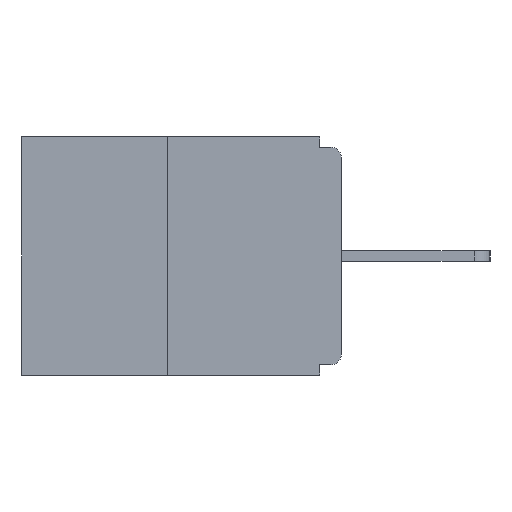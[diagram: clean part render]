
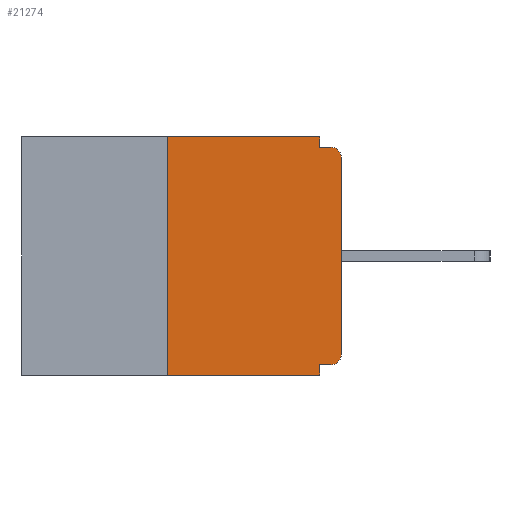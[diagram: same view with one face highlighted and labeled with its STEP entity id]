
A CAD part, left-side view. The second image highlights one B-rep face of the part: STEP entity #21274.
In plain terms, the highlighted planar face has unit normal (-1, 0, 0).
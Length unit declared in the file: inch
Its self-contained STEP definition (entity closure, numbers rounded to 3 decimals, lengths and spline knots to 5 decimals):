
#655 = VERTEX_POINT ( 'NONE', #2800 ) ;
#684 = LINE ( 'NONE', #15329, #5969 ) ;
#745 = LINE ( 'NONE', #10344, #6030 ) ;
#1100 = ORIENTED_EDGE ( 'NONE', *, *, #23193, .F. ) ;
#1425 = ORIENTED_EDGE ( 'NONE', *, *, #22198, .T. ) ;
#1452 = PLANE ( 'NONE',  #21890 ) ;
#1503 = VECTOR ( 'NONE', #11871, 39.37008 ) ;
#1712 = DIRECTION ( 'NONE',  ( 0., -1., 0. ) ) ;
#1864 = DIRECTION ( 'NONE',  ( 0., -1., 0. ) ) ;
#2619 = VECTOR ( 'NONE', #17987, 39.37008 ) ;
#2800 = CARTESIAN_POINT ( 'NONE',  ( 0., 0.25, 0. ) ) ;
#3467 = DIRECTION ( 'NONE',  ( 0., 0., -1. ) ) ;
#3542 = VERTEX_POINT ( 'NONE', #7040 ) ;
#3917 = FACE_OUTER_BOUND ( 'NONE', #17528, .T. ) ;
#4743 = VERTEX_POINT ( 'NONE', #6163 ) ;
#4797 = VECTOR ( 'NONE', #16912, 39.37008 ) ;
#4858 = CARTESIAN_POINT ( 'NONE',  ( 0., 0.031, -0.343 ) ) ;
#4873 = CARTESIAN_POINT ( 'NONE',  ( 0., 0.46, -0.343 ) ) ;
#5411 = EDGE_CURVE ( 'NONE', #11106, #9800, #15516, .T. ) ;
#5480 = VECTOR ( 'NONE', #18613, 39.37008 ) ;
#5969 = VECTOR ( 'NONE', #1712, 39.37008 ) ;
#6030 = VECTOR ( 'NONE', #12242, 39.37008 ) ;
#6163 = CARTESIAN_POINT ( 'NONE',  ( 0., 0.25, -0.343 ) ) ;
#6356 = LINE ( 'NONE', #24986, #11791 ) ;
#7040 = CARTESIAN_POINT ( 'NONE',  ( 0., 0.031, -0.328 ) ) ;
#7148 = VERTEX_POINT ( 'NONE', #17537 ) ;
#7246 = CARTESIAN_POINT ( 'NONE',  ( 0., 0.25, 0. ) ) ;
#7995 = CARTESIAN_POINT ( 'NONE',  ( 0., 0., -0.328 ) ) ;
#8064 = EDGE_CURVE ( 'NONE', #21727, #9620, #14606, .T. ) ;
#8852 = DIRECTION ( 'NONE',  ( 0., -1., 0. ) ) ;
#9620 = VERTEX_POINT ( 'NONE', #10226 ) ;
#9800 = VERTEX_POINT ( 'NONE', #14513 ) ;
#10187 = CARTESIAN_POINT ( 'NONE',  ( 0., 0.015, -0.03 ) ) ;
#10226 = CARTESIAN_POINT ( 'NONE',  ( 0., 0., -0.313 ) ) ;
#10344 = CARTESIAN_POINT ( 'NONE',  ( 0., 0.031, -0.343 ) ) ;
#10692 = EDGE_CURVE ( 'NONE', #14422, #9800, #6356, .T. ) ;
#10988 = CARTESIAN_POINT ( 'NONE',  ( 0., 0.015, -0.313 ) ) ;
#11106 = VERTEX_POINT ( 'NONE', #12963 ) ;
#11791 = VECTOR ( 'NONE', #1864, 39.37008 ) ;
#11871 = DIRECTION ( 'NONE',  ( 0., 1., 0. ) ) ;
#11885 = LINE ( 'NONE', #12737, #5480 ) ;
#12081 = DIRECTION ( 'NONE',  ( 0., 0., -1. ) ) ;
#12242 = DIRECTION ( 'NONE',  ( 0., 0., -1. ) ) ;
#12737 = CARTESIAN_POINT ( 'NONE',  ( 0., 0.031, 0. ) ) ;
#12838 = VERTEX_POINT ( 'NONE', #4858 ) ;
#12882 = DIRECTION ( 'NONE',  ( 0., 0., -1. ) ) ;
#12963 = CARTESIAN_POINT ( 'NONE',  ( 0., 0., -0.03 ) ) ;
#13065 = ORIENTED_EDGE ( 'NONE', *, *, #10692, .F. ) ;
#14422 = VERTEX_POINT ( 'NONE', #15964 ) ;
#14513 = CARTESIAN_POINT ( 'NONE',  ( 0., 0.015, -0.015 ) ) ;
#14535 = ORIENTED_EDGE ( 'NONE', *, *, #18038, .F. ) ;
#14554 = CARTESIAN_POINT ( 'NONE',  ( 0., 0.015, -0.328 ) ) ;
#14606 = CIRCLE ( 'NONE', #23409, 0.015 ) ;
#15090 = DIRECTION ( 'NONE',  ( 1., 0., 0. ) ) ;
#15329 = CARTESIAN_POINT ( 'NONE',  ( 0., 0.46, 0. ) ) ;
#15516 = CIRCLE ( 'NONE', #21309, 0.015 ) ;
#15785 = EDGE_CURVE ( 'NONE', #21727, #3542, #22105, .T. ) ;
#15964 = CARTESIAN_POINT ( 'NONE',  ( 0., 0.031, -0.015 ) ) ;
#16048 = CARTESIAN_POINT ( 'NONE',  ( 0., 0., 0. ) ) ;
#16735 = EDGE_CURVE ( 'NONE', #7148, #14422, #11885, .T. ) ;
#16912 = DIRECTION ( 'NONE',  ( 0., 0., 1. ) ) ;
#17528 = EDGE_LOOP ( 'NONE', ( #1100, #17852, #24103, #14535, #20239, #20838, #1425, #22032, #13065, #18772 ) ) ;
#17537 = CARTESIAN_POINT ( 'NONE',  ( 0., 0.031, 0. ) ) ;
#17852 = ORIENTED_EDGE ( 'NONE', *, *, #21861, .F. ) ;
#17987 = DIRECTION ( 'NONE',  ( 0., 0., 1. ) ) ;
#18038 = EDGE_CURVE ( 'NONE', #3542, #12838, #745, .T. ) ;
#18613 = DIRECTION ( 'NONE',  ( 0., 0., -1. ) ) ;
#18772 = ORIENTED_EDGE ( 'NONE', *, *, #16735, .F. ) ;
#18877 = CARTESIAN_POINT ( 'NONE',  ( 0., 0.46, 0. ) ) ;
#19676 = VECTOR ( 'NONE', #8852, 39.37008 ) ;
#20199 = LINE ( 'NONE', #7246, #4797 ) ;
#20239 = ORIENTED_EDGE ( 'NONE', *, *, #15785, .F. ) ;
#20597 = EDGE_CURVE ( 'NONE', #4743, #12838, #24725, .T. ) ;
#20838 = ORIENTED_EDGE ( 'NONE', *, *, #8064, .T. ) ;
#21274 = ADVANCED_FACE ( 'NONE', ( #3917 ), #1452, .F. ) ;
#21309 = AXIS2_PLACEMENT_3D ( 'NONE', #10187, #23505, #12081 ) ;
#21727 = VERTEX_POINT ( 'NONE', #14554 ) ;
#21861 = EDGE_CURVE ( 'NONE', #4743, #655, #20199, .T. ) ;
#21890 = AXIS2_PLACEMENT_3D ( 'NONE', #18877, #15090, #3467 ) ;
#22032 = ORIENTED_EDGE ( 'NONE', *, *, #5411, .T. ) ;
#22105 = LINE ( 'NONE', #7995, #1503 ) ;
#22198 = EDGE_CURVE ( 'NONE', #9620, #11106, #24936, .T. ) ;
#23193 = EDGE_CURVE ( 'NONE', #655, #7148, #684, .T. ) ;
#23409 = AXIS2_PLACEMENT_3D ( 'NONE', #10988, #24328, #12882 ) ;
#23505 = DIRECTION ( 'NONE',  ( -1., 0., 0. ) ) ;
#24103 = ORIENTED_EDGE ( 'NONE', *, *, #20597, .T. ) ;
#24328 = DIRECTION ( 'NONE',  ( -1., 0., 0. ) ) ;
#24725 = LINE ( 'NONE', #4873, #19676 ) ;
#24936 = LINE ( 'NONE', #16048, #2619 ) ;
#24986 = CARTESIAN_POINT ( 'NONE',  ( 0., 0., -0.015 ) ) ;
